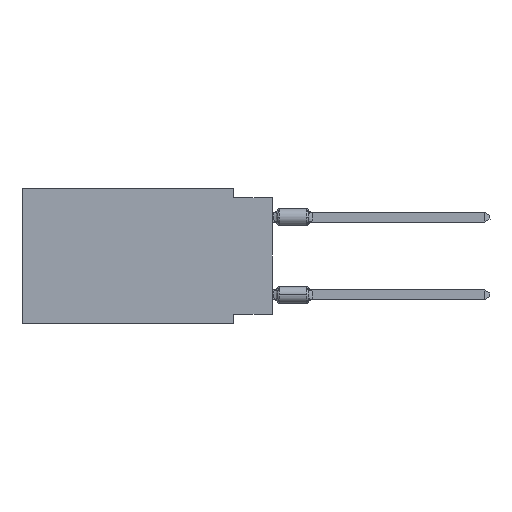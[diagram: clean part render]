
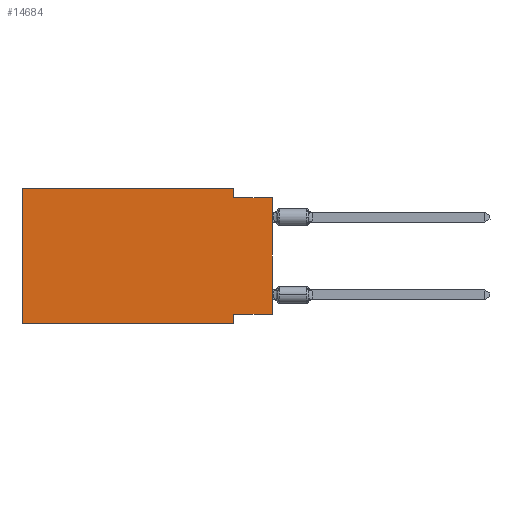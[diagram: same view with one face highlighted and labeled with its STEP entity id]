
A CAD part, left-side view. The second image highlights one B-rep face of the part: STEP entity #14684.
In plain terms, the highlighted planar face has unit normal (-1, 0, 0).
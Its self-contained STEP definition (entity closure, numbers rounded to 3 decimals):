
#546 = VERTEX_POINT ( 'NONE', #17329 ) ;
#1075 = LINE ( 'NONE', #15993, #10441 ) ;
#1485 = CARTESIAN_POINT ( 'NONE',  ( 0., 0., 0. ) ) ;
#1784 = CARTESIAN_POINT ( 'NONE',  ( 0., 16.383, 0. ) ) ;
#2856 = CARTESIAN_POINT ( 'NONE',  ( 0., 16.383, 0. ) ) ;
#3003 = ORIENTED_EDGE ( 'NONE', *, *, #9249, .F. ) ;
#3095 = ORIENTED_EDGE ( 'NONE', *, *, #8263, .F. ) ;
#3122 = DIRECTION ( 'NONE',  ( 0., -1., 0. ) ) ;
#3214 = LINE ( 'NONE', #9284, #18017 ) ;
#3460 = CARTESIAN_POINT ( 'NONE',  ( 0., 0., -0.635 ) ) ;
#3810 = EDGE_LOOP ( 'NONE', ( #18806, #18739, #3003, #3095, #13999, #19408, #8616, #14365 ) ) ;
#4475 = CARTESIAN_POINT ( 'NONE',  ( 0., 0., -8.255 ) ) ;
#4684 = VERTEX_POINT ( 'NONE', #12777 ) ;
#4731 = CARTESIAN_POINT ( 'NONE',  ( 0., 0., -0.635 ) ) ;
#4957 = LINE ( 'NONE', #11023, #13132 ) ;
#5903 = AXIS2_PLACEMENT_3D ( 'NONE', #1784, #12535, #18611 ) ;
#7167 = LINE ( 'NONE', #4475, #8638 ) ;
#8059 = FACE_OUTER_BOUND ( 'NONE', #3810, .T. ) ;
#8263 = EDGE_CURVE ( 'NONE', #14036, #18625, #3214, .T. ) ;
#8429 = DIRECTION ( 'NONE',  ( 0., -1., 0. ) ) ;
#8599 = VECTOR ( 'NONE', #10633, 1000. ) ;
#8616 = ORIENTED_EDGE ( 'NONE', *, *, #18073, .F. ) ;
#8638 = VECTOR ( 'NONE', #12045, 1000. ) ;
#9010 = VECTOR ( 'NONE', #12623, 1000. ) ;
#9249 = EDGE_CURVE ( 'NONE', #18625, #19588, #9835, .T. ) ;
#9284 = CARTESIAN_POINT ( 'NONE',  ( 0., 16.383, 0. ) ) ;
#9835 = LINE ( 'NONE', #15803, #9010 ) ;
#10160 = EDGE_CURVE ( 'NONE', #4684, #17340, #7167, .T. ) ;
#10441 = VECTOR ( 'NONE', #8429, 1000. ) ;
#10487 = DIRECTION ( 'NONE',  ( 0., 0., -1. ) ) ;
#10633 = DIRECTION ( 'NONE',  ( 0., 0., 1. ) ) ;
#11023 = CARTESIAN_POINT ( 'NONE',  ( 0., 16.383, 0. ) ) ;
#11789 = CARTESIAN_POINT ( 'NONE',  ( 0., 2.54, -8.89 ) ) ;
#11988 = CARTESIAN_POINT ( 'NONE',  ( 0., 2.54, -8.89 ) ) ;
#12045 = DIRECTION ( 'NONE',  ( 0., 1., 0. ) ) ;
#12507 = EDGE_CURVE ( 'NONE', #546, #14036, #4957, .T. ) ;
#12535 = DIRECTION ( 'NONE',  ( 1., 0., 0. ) ) ;
#12623 = DIRECTION ( 'NONE',  ( 0., 0., -1. ) ) ;
#12777 = CARTESIAN_POINT ( 'NONE',  ( 0., 0., -8.255 ) ) ;
#13132 = VECTOR ( 'NONE', #17596, 1000. ) ;
#13625 = CARTESIAN_POINT ( 'NONE',  ( 0., 2.54, 0. ) ) ;
#13751 = EDGE_CURVE ( 'NONE', #19588, #19029, #17099, .T. ) ;
#13999 = ORIENTED_EDGE ( 'NONE', *, *, #12507, .F. ) ;
#14036 = VERTEX_POINT ( 'NONE', #2856 ) ;
#14291 = VECTOR ( 'NONE', #10487, 1000. ) ;
#14365 = ORIENTED_EDGE ( 'NONE', *, *, #10160, .F. ) ;
#14684 = ADVANCED_FACE ( 'NONE', ( #8059 ), #18507, .F. ) ;
#15074 = LINE ( 'NONE', #11789, #14291 ) ;
#15598 = DIRECTION ( 'NONE',  ( 0., -1., 0. ) ) ;
#15803 = CARTESIAN_POINT ( 'NONE',  ( 0., 2.54, 0. ) ) ;
#15993 = CARTESIAN_POINT ( 'NONE',  ( 0., 16.383, -8.89 ) ) ;
#16373 = EDGE_CURVE ( 'NONE', #546, #18127, #1075, .T. ) ;
#16506 = CARTESIAN_POINT ( 'NONE',  ( 0., 2.54, -8.255 ) ) ;
#16797 = LINE ( 'NONE', #1485, #8599 ) ;
#17099 = LINE ( 'NONE', #3460, #18040 ) ;
#17329 = CARTESIAN_POINT ( 'NONE',  ( 0., 16.383, -8.89 ) ) ;
#17340 = VERTEX_POINT ( 'NONE', #16506 ) ;
#17596 = DIRECTION ( 'NONE',  ( 0., 0., 1. ) ) ;
#18017 = VECTOR ( 'NONE', #3122, 1000. ) ;
#18040 = VECTOR ( 'NONE', #15598, 1000. ) ;
#18073 = EDGE_CURVE ( 'NONE', #17340, #18127, #15074, .T. ) ;
#18127 = VERTEX_POINT ( 'NONE', #11988 ) ;
#18507 = PLANE ( 'NONE',  #5903 ) ;
#18595 = EDGE_CURVE ( 'NONE', #4684, #19029, #16797, .T. ) ;
#18611 = DIRECTION ( 'NONE',  ( 0., 0., -1. ) ) ;
#18625 = VERTEX_POINT ( 'NONE', #13625 ) ;
#18644 = CARTESIAN_POINT ( 'NONE',  ( 0., 2.54, -0.635 ) ) ;
#18739 = ORIENTED_EDGE ( 'NONE', *, *, #13751, .F. ) ;
#18806 = ORIENTED_EDGE ( 'NONE', *, *, #18595, .T. ) ;
#19029 = VERTEX_POINT ( 'NONE', #4731 ) ;
#19408 = ORIENTED_EDGE ( 'NONE', *, *, #16373, .T. ) ;
#19588 = VERTEX_POINT ( 'NONE', #18644 ) ;
